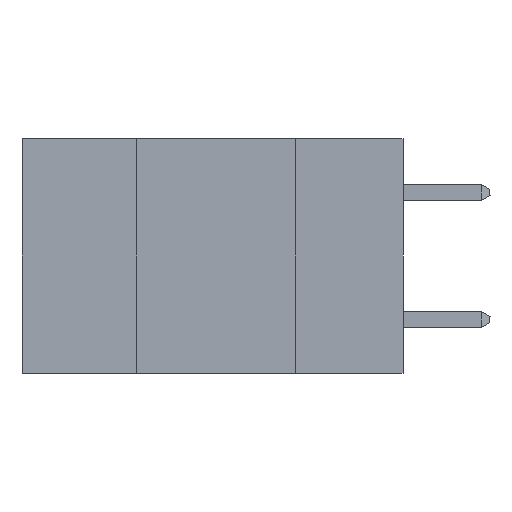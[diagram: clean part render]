
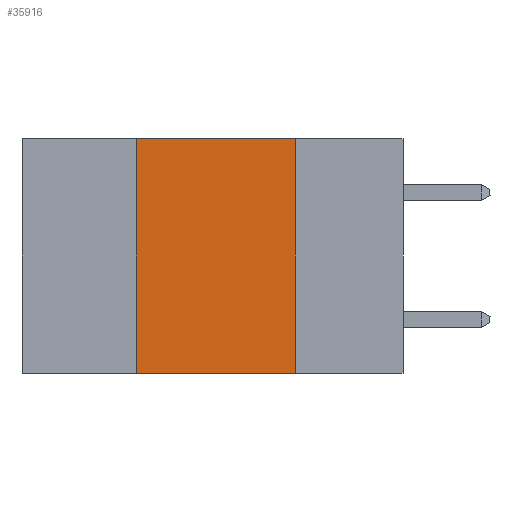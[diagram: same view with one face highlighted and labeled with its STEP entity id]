
A CAD part, left-side view. The second image highlights one B-rep face of the part: STEP entity #35916.
In plain terms, the highlighted planar face has unit normal (-1, 0, 0).
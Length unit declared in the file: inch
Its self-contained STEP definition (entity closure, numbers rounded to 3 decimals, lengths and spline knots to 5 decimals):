
#427 = ORIENTED_EDGE ( 'NONE', *, *, #43281, .T. ) ;
#592 = ORIENTED_EDGE ( 'NONE', *, *, #25176, .F. ) ;
#2146 = VECTOR ( 'NONE', #17850, 39.37008 ) ;
#2561 = VECTOR ( 'NONE', #29358, 39.37008 ) ;
#3243 = CARTESIAN_POINT ( 'NONE',  ( 0., 0.6, 0. ) ) ;
#3403 = DIRECTION ( 'NONE',  ( 0., 0., -1. ) ) ;
#3920 = FACE_OUTER_BOUND ( 'NONE', #28700, .T. ) ;
#4972 = CARTESIAN_POINT ( 'NONE',  ( 0., 0.42, 0. ) ) ;
#10528 = CARTESIAN_POINT ( 'NONE',  ( 0., 0.6, 0. ) ) ;
#10976 = AXIS2_PLACEMENT_3D ( 'NONE', #3243, #45320, #3403 ) ;
#11493 = LINE ( 'NONE', #10528, #2146 ) ;
#13685 = DIRECTION ( 'NONE',  ( 0., 0., 1. ) ) ;
#14360 = VERTEX_POINT ( 'NONE', #39812 ) ;
#16100 = CARTESIAN_POINT ( 'NONE',  ( 0., 0.17, -0.37 ) ) ;
#16562 = LINE ( 'NONE', #21050, #30890 ) ;
#16871 = PLANE ( 'NONE',  #10976 ) ;
#17850 = DIRECTION ( 'NONE',  ( 0., -1., 0. ) ) ;
#18361 = CARTESIAN_POINT ( 'NONE',  ( 0., 0.6, -0.37 ) ) ;
#19676 = VECTOR ( 'NONE', #39593, 39.37008 ) ;
#21050 = CARTESIAN_POINT ( 'NONE',  ( 0., 0.42, 0. ) ) ;
#22320 = LINE ( 'NONE', #36312, #2561 ) ;
#25176 = EDGE_CURVE ( 'NONE', #14360, #41003, #22320, .T. ) ;
#28271 = VERTEX_POINT ( 'NONE', #33185 ) ;
#28700 = EDGE_LOOP ( 'NONE', ( #592, #30704, #37495, #427 ) ) ;
#29358 = DIRECTION ( 'NONE',  ( 0., 0., -1. ) ) ;
#30704 = ORIENTED_EDGE ( 'NONE', *, *, #34743, .F. ) ;
#30890 = VECTOR ( 'NONE', #13685, 39.37008 ) ;
#33185 = CARTESIAN_POINT ( 'NONE',  ( 0., 0.42, -0.37 ) ) ;
#34743 = EDGE_CURVE ( 'NONE', #40221, #14360, #11493, .T. ) ;
#35284 = EDGE_CURVE ( 'NONE', #28271, #40221, #16562, .T. ) ;
#35916 = ADVANCED_FACE ( 'NONE', ( #3920 ), #16871, .F. ) ;
#36312 = CARTESIAN_POINT ( 'NONE',  ( 0., 0.17, 0. ) ) ;
#37495 = ORIENTED_EDGE ( 'NONE', *, *, #35284, .F. ) ;
#38396 = LINE ( 'NONE', #18361, #19676 ) ;
#39593 = DIRECTION ( 'NONE',  ( 0., -1., 0. ) ) ;
#39812 = CARTESIAN_POINT ( 'NONE',  ( 0., 0.17, 0. ) ) ;
#40221 = VERTEX_POINT ( 'NONE', #4972 ) ;
#41003 = VERTEX_POINT ( 'NONE', #16100 ) ;
#43281 = EDGE_CURVE ( 'NONE', #28271, #41003, #38396, .T. ) ;
#45320 = DIRECTION ( 'NONE',  ( 1., 0., 0. ) ) ;
